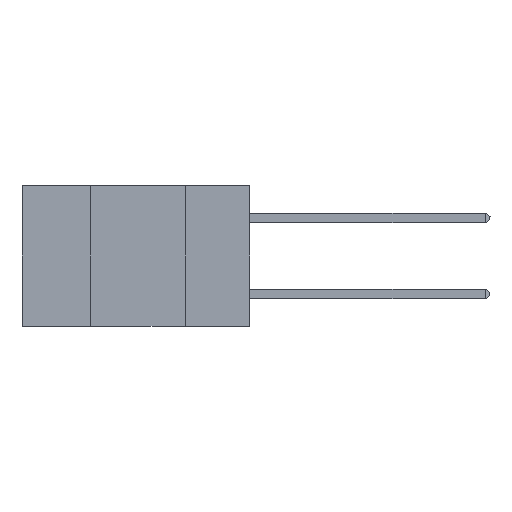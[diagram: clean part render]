
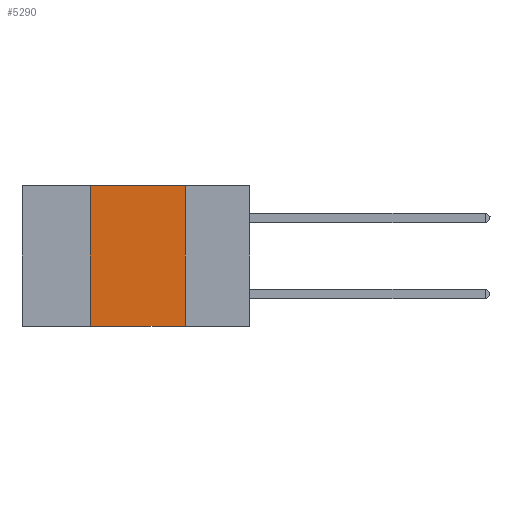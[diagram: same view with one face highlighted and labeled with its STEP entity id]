
A CAD part, left-side view. The second image highlights one B-rep face of the part: STEP entity #5290.
In plain terms, the highlighted planar face has unit normal (-1, 0, 0).
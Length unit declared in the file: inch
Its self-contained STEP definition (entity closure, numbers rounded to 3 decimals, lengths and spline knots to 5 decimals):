
#687 = LINE ( 'NONE', #12616, #11831 ) ;
#719 = EDGE_CURVE ( 'NONE', #7491, #2434, #687, .T. ) ;
#748 = DIRECTION ( 'NONE',  ( 0., -1., 0. ) ) ;
#869 = VECTOR ( 'NONE', #8748, 39.37008 ) ;
#1128 = PLANE ( 'NONE',  #12065 ) ;
#1388 = DIRECTION ( 'NONE',  ( 0., 0., -1. ) ) ;
#1717 = CARTESIAN_POINT ( 'NONE',  ( 0., 0.17, -0.37 ) ) ;
#2434 = VERTEX_POINT ( 'NONE', #1717 ) ;
#3204 = CARTESIAN_POINT ( 'NONE',  ( 0., 0.17, 0. ) ) ;
#3674 = VERTEX_POINT ( 'NONE', #6824 ) ;
#4068 = VECTOR ( 'NONE', #748, 39.37008 ) ;
#4362 = DIRECTION ( 'NONE',  ( 1., 0., 0. ) ) ;
#4789 = VERTEX_POINT ( 'NONE', #6590 ) ;
#4941 = ORIENTED_EDGE ( 'NONE', *, *, #8198, .F. ) ;
#5054 = ORIENTED_EDGE ( 'NONE', *, *, #9283, .F. ) ;
#5290 = ADVANCED_FACE ( 'NONE', ( #9063 ), #1128, .F. ) ;
#5730 = ORIENTED_EDGE ( 'NONE', *, *, #9545, .T. ) ;
#6269 = LINE ( 'NONE', #8765, #869 ) ;
#6590 = CARTESIAN_POINT ( 'NONE',  ( 0., 0.42, 0. ) ) ;
#6824 = CARTESIAN_POINT ( 'NONE',  ( 0., 0.42, -0.37 ) ) ;
#7174 = CARTESIAN_POINT ( 'NONE',  ( 0., 0.6, -0.37 ) ) ;
#7226 = DIRECTION ( 'NONE',  ( 0., 0., -1. ) ) ;
#7384 = LINE ( 'NONE', #7823, #7710 ) ;
#7491 = VERTEX_POINT ( 'NONE', #3204 ) ;
#7710 = VECTOR ( 'NONE', #8852, 39.37008 ) ;
#7823 = CARTESIAN_POINT ( 'NONE',  ( 0., 0.6, 0. ) ) ;
#7839 = ORIENTED_EDGE ( 'NONE', *, *, #719, .F. ) ;
#8198 = EDGE_CURVE ( 'NONE', #3674, #4789, #6269, .T. ) ;
#8748 = DIRECTION ( 'NONE',  ( 0., 0., 1. ) ) ;
#8765 = CARTESIAN_POINT ( 'NONE',  ( 0., 0.42, 0. ) ) ;
#8852 = DIRECTION ( 'NONE',  ( 0., -1., 0. ) ) ;
#9063 = FACE_OUTER_BOUND ( 'NONE', #12755, .T. ) ;
#9283 = EDGE_CURVE ( 'NONE', #4789, #7491, #7384, .T. ) ;
#9545 = EDGE_CURVE ( 'NONE', #3674, #2434, #11969, .T. ) ;
#11831 = VECTOR ( 'NONE', #7226, 39.37008 ) ;
#11969 = LINE ( 'NONE', #7174, #4068 ) ;
#12065 = AXIS2_PLACEMENT_3D ( 'NONE', #12865, #4362, #1388 ) ;
#12616 = CARTESIAN_POINT ( 'NONE',  ( 0., 0.17, 0. ) ) ;
#12755 = EDGE_LOOP ( 'NONE', ( #7839, #5054, #4941, #5730 ) ) ;
#12865 = CARTESIAN_POINT ( 'NONE',  ( 0., 0.6, 0. ) ) ;
